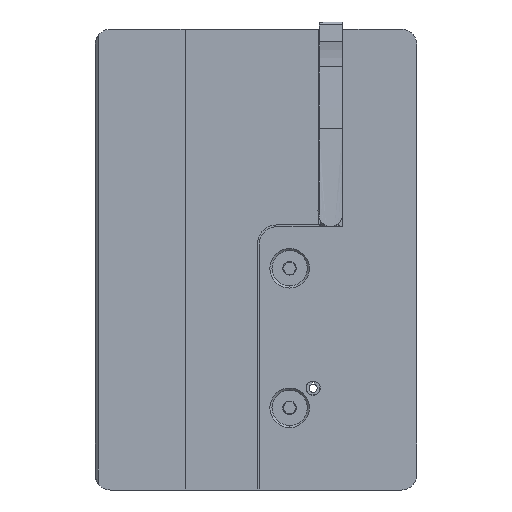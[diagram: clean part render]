
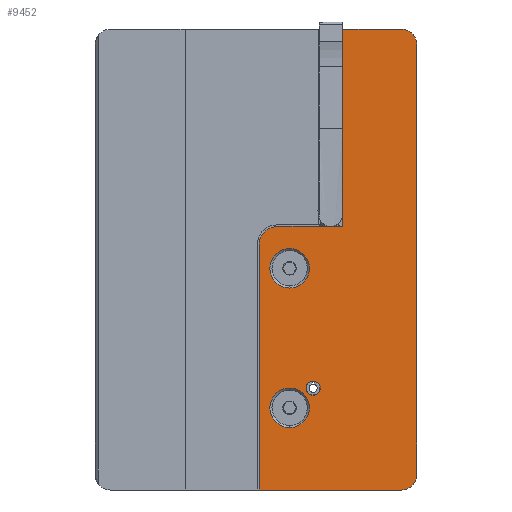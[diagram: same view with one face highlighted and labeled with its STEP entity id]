
A CAD part, left-side view. The second image highlights one B-rep face of the part: STEP entity #9452.
In plain terms, the highlighted planar face has unit normal (-1, 0, 0).
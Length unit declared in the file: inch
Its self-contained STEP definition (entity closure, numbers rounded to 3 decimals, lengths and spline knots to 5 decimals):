
#277 = CARTESIAN_POINT ( 'NONE',  ( -0.5, -0.41732, 0.025 ) ) ;
#498 = AXIS2_PLACEMENT_3D ( 'NONE', #7511, #19767, #10806 ) ;
#588 = EDGE_CURVE ( 'NONE', #7306, #6336, #9116, .T. ) ;
#1008 = CIRCLE ( 'NONE', #19829, 0.1 ) ;
#1064 = EDGE_CURVE ( 'NONE', #22464, #15260, #9641, .T. ) ;
#1150 = CARTESIAN_POINT ( 'NONE',  ( -0.5, 0.33268, -1.34272 ) ) ;
#1222 = CARTESIAN_POINT ( 'NONE',  ( -0.5, -0.51732, -2.85894 ) ) ;
#1831 = ORIENTED_EDGE ( 'NONE', *, *, #11971, .F. ) ;
#1925 = DIRECTION ( 'NONE',  ( -1., 0., 0. ) ) ;
#2478 = DIRECTION ( 'NONE',  ( 0., 0., 1. ) ) ;
#2717 = CARTESIAN_POINT ( 'NONE',  ( -0.5, 0.17531, -2.32502 ) ) ;
#2830 = PLANE ( 'NONE',  #10038 ) ;
#3038 = DIRECTION ( 'NONE',  ( -1., 0., 0. ) ) ;
#3093 = CARTESIAN_POINT ( 'NONE',  ( -0.5, 0.41187, -1.195 ) ) ;
#3456 = VERTEX_POINT ( 'NONE', #22065 ) ;
#3533 = EDGE_CURVE ( 'NONE', #13325, #19146, #14831, .T. ) ;
#3816 = DIRECTION ( 'NONE',  ( 0., 0., -1. ) ) ;
#3877 = CARTESIAN_POINT ( 'NONE',  ( -0.5, -0.51732, 0.125 ) ) ;
#4134 = CARTESIAN_POINT ( 'NONE',  ( -0.5, 0.53687, -1.195 ) ) ;
#4220 = DIRECTION ( 'NONE',  ( 0., 0., -1. ) ) ;
#4461 = ORIENTED_EDGE ( 'NONE', *, *, #13157, .F. ) ;
#4485 = DIRECTION ( 'NONE',  ( -1., 0., 0. ) ) ;
#4728 = ORIENTED_EDGE ( 'NONE', *, *, #16448, .F. ) ;
#5050 = VECTOR ( 'NONE', #4220, 39.37008 ) ;
#5121 = CARTESIAN_POINT ( 'NONE',  ( -0.5, -0.02313, 0.125 ) ) ;
#5163 = CARTESIAN_POINT ( 'NONE',  ( -0.5, 0.53687, -1.32 ) ) ;
#5471 = CARTESIAN_POINT ( 'NONE',  ( -0.5, -0.51732, 0.025 ) ) ;
#5515 = EDGE_CURVE ( 'NONE', #19146, #13325, #7239, .T. ) ;
#5532 = CARTESIAN_POINT ( 'NONE',  ( -0.5, 0.17531, -2.27752 ) ) ;
#5645 = DIRECTION ( 'NONE',  ( -1., 0., 0. ) ) ;
#5661 = AXIS2_PLACEMENT_3D ( 'NONE', #5532, #5645, #12807 ) ;
#5664 = LINE ( 'NONE', #12823, #6266 ) ;
#5711 = FACE_OUTER_BOUND ( 'NONE', #12936, .T. ) ;
#5741 = VERTEX_POINT ( 'NONE', #17261 ) ;
#6068 = VECTOR ( 'NONE', #6070, 39.37008 ) ;
#6070 = DIRECTION ( 'NONE',  ( 0., 1., 0. ) ) ;
#6266 = VECTOR ( 'NONE', #16481, 39.37008 ) ;
#6329 = DIRECTION ( 'NONE',  ( 0., 0., 1. ) ) ;
#6336 = VERTEX_POINT ( 'NONE', #1222 ) ;
#6407 = VERTEX_POINT ( 'NONE', #5471 ) ;
#6463 = FACE_BOUND ( 'NONE', #16546, .T. ) ;
#6827 = CIRCLE ( 'NONE', #8323, 0.13228 ) ;
#6839 = DIRECTION ( 'NONE',  ( -1., 0., 0. ) ) ;
#7117 = CIRCLE ( 'NONE', #19930, 0.0475 ) ;
#7217 = CARTESIAN_POINT ( 'NONE',  ( -0.5, 0.33268, -2.409 ) ) ;
#7239 = CIRCLE ( 'NONE', #498, 0.13228 ) ;
#7306 = VERTEX_POINT ( 'NONE', #19699 ) ;
#7511 = CARTESIAN_POINT ( 'NONE',  ( -0.5, 0.33268, -1.475 ) ) ;
#8208 = CARTESIAN_POINT ( 'NONE',  ( -0.5, 0.33268, -1.475 ) ) ;
#8210 = VERTEX_POINT ( 'NONE', #20801 ) ;
#8323 = AXIS2_PLACEMENT_3D ( 'NONE', #7217, #1925, #9099 ) ;
#8377 = EDGE_LOOP ( 'NONE', ( #10103, #8920 ) ) ;
#8915 = CARTESIAN_POINT ( 'NONE',  ( -0.5, -0.23642, 0.125 ) ) ;
#8920 = ORIENTED_EDGE ( 'NONE', *, *, #3533, .F. ) ;
#8970 = DIRECTION ( 'NONE',  ( 0., 0., -1. ) ) ;
#9099 = DIRECTION ( 'NONE',  ( 0., 0., 1. ) ) ;
#9116 = CIRCLE ( 'NONE', #11008, 0.1 ) ;
#9452 = ADVANCED_FACE ( 'NONE', ( #5711, #6463, #16952, #21830 ), #2830, .F. ) ;
#9533 = ORIENTED_EDGE ( 'NONE', *, *, #11877, .T. ) ;
#9641 = LINE ( 'NONE', #4134, #13998 ) ;
#10003 = DIRECTION ( 'NONE',  ( 1., 0., 0. ) ) ;
#10038 = AXIS2_PLACEMENT_3D ( 'NONE', #15413, #10003, #22475 ) ;
#10048 = CARTESIAN_POINT ( 'NONE',  ( -0.5, -0.02313, -1.195 ) ) ;
#10103 = ORIENTED_EDGE ( 'NONE', *, *, #5515, .F. ) ;
#10136 = CARTESIAN_POINT ( 'NONE',  ( -0.5, 0.17531, -2.23002 ) ) ;
#10483 = ORIENTED_EDGE ( 'NONE', *, *, #12620, .T. ) ;
#10503 = LINE ( 'NONE', #5121, #22251 ) ;
#10806 = DIRECTION ( 'NONE',  ( 0., 0., 1. ) ) ;
#11008 = AXIS2_PLACEMENT_3D ( 'NONE', #21718, #17941, #3816 ) ;
#11050 = LINE ( 'NONE', #3877, #5050 ) ;
#11057 = CARTESIAN_POINT ( 'NONE',  ( -0.5, 0.33268, -2.409 ) ) ;
#11141 = ORIENTED_EDGE ( 'NONE', *, *, #19686, .F. ) ;
#11406 = CARTESIAN_POINT ( 'NONE',  ( -0.5, -0.41732, 0.125 ) ) ;
#11481 = LINE ( 'NONE', #22310, #6068 ) ;
#11877 = EDGE_CURVE ( 'NONE', #22464, #17074, #18717, .T. ) ;
#11962 = EDGE_LOOP ( 'NONE', ( #15218, #17187 ) ) ;
#11971 = EDGE_CURVE ( 'NONE', #14764, #17074, #5664, .T. ) ;
#12027 = CIRCLE ( 'NONE', #5661, 0.0475 ) ;
#12370 = DIRECTION ( 'NONE',  ( 0., 0., 1. ) ) ;
#12620 = EDGE_CURVE ( 'NONE', #6407, #19960, #1008, .T. ) ;
#12807 = DIRECTION ( 'NONE',  ( 0., 0., 1. ) ) ;
#12823 = CARTESIAN_POINT ( 'NONE',  ( -0.5, 0.53687, -2.95894 ) ) ;
#12936 = EDGE_LOOP ( 'NONE', ( #20408, #21077, #4461, #10483, #16747, #11141, #20574, #9533, #1831 ) ) ;
#12940 = AXIS2_PLACEMENT_3D ( 'NONE', #8208, #3038, #6329 ) ;
#13065 = DIRECTION ( 'NONE',  ( 0., -1., 0. ) ) ;
#13157 = EDGE_CURVE ( 'NONE', #6407, #6336, #11050, .T. ) ;
#13325 = VERTEX_POINT ( 'NONE', #15236 ) ;
#13397 = AXIS2_PLACEMENT_3D ( 'NONE', #22236, #22018, #18123 ) ;
#13901 = VERTEX_POINT ( 'NONE', #10136 ) ;
#13998 = VECTOR ( 'NONE', #13065, 39.37008 ) ;
#14764 = VERTEX_POINT ( 'NONE', #15451 ) ;
#14831 = CIRCLE ( 'NONE', #12940, 0.13228 ) ;
#15078 = CIRCLE ( 'NONE', #19208, 0.13228 ) ;
#15218 = ORIENTED_EDGE ( 'NONE', *, *, #21934, .F. ) ;
#15236 = CARTESIAN_POINT ( 'NONE',  ( -0.5, 0.33268, -1.60728 ) ) ;
#15260 = VERTEX_POINT ( 'NONE', #10048 ) ;
#15413 = CARTESIAN_POINT ( 'NONE',  ( -0.5, 0., 0. ) ) ;
#15451 = CARTESIAN_POINT ( 'NONE',  ( -0.5, 0.53687, -2.95894 ) ) ;
#15996 = EDGE_CURVE ( 'NONE', #18796, #13901, #7117, .T. ) ;
#16095 = DIRECTION ( 'NONE',  ( 0., 1., 0. ) ) ;
#16448 = EDGE_CURVE ( 'NONE', #13901, #18796, #12027, .T. ) ;
#16481 = DIRECTION ( 'NONE',  ( 0., 0., 1. ) ) ;
#16546 = EDGE_LOOP ( 'NONE', ( #4728, #19377 ) ) ;
#16644 = VECTOR ( 'NONE', #16095, 39.37008 ) ;
#16747 = ORIENTED_EDGE ( 'NONE', *, *, #20383, .T. ) ;
#16952 = FACE_BOUND ( 'NONE', #11962, .T. ) ;
#17074 = VERTEX_POINT ( 'NONE', #5163 ) ;
#17187 = ORIENTED_EDGE ( 'NONE', *, *, #18343, .F. ) ;
#17261 = CARTESIAN_POINT ( 'NONE',  ( -0.5, -0.02313, 0.125 ) ) ;
#17744 = LINE ( 'NONE', #8915, #16644 ) ;
#17925 = DIRECTION ( 'NONE',  ( -1., 0., 0. ) ) ;
#17941 = DIRECTION ( 'NONE',  ( -1., 0., 0. ) ) ;
#18123 = DIRECTION ( 'NONE',  ( 0., 0., -1. ) ) ;
#18343 = EDGE_CURVE ( 'NONE', #8210, #3456, #15078, .T. ) ;
#18717 = CIRCLE ( 'NONE', #13397, 0.125 ) ;
#18796 = VERTEX_POINT ( 'NONE', #2717 ) ;
#19146 = VERTEX_POINT ( 'NONE', #1150 ) ;
#19208 = AXIS2_PLACEMENT_3D ( 'NONE', #11057, #6839, #12370 ) ;
#19377 = ORIENTED_EDGE ( 'NONE', *, *, #15996, .F. ) ;
#19686 = EDGE_CURVE ( 'NONE', #15260, #5741, #10503, .T. ) ;
#19699 = CARTESIAN_POINT ( 'NONE',  ( -0.5, -0.41732, -2.95894 ) ) ;
#19767 = DIRECTION ( 'NONE',  ( -1., 0., 0. ) ) ;
#19829 = AXIS2_PLACEMENT_3D ( 'NONE', #277, #17925, #8970 ) ;
#19930 = AXIS2_PLACEMENT_3D ( 'NONE', #20603, #4485, #2478 ) ;
#19960 = VERTEX_POINT ( 'NONE', #11406 ) ;
#20383 = EDGE_CURVE ( 'NONE', #19960, #5741, #17744, .T. ) ;
#20408 = ORIENTED_EDGE ( 'NONE', *, *, #21526, .F. ) ;
#20574 = ORIENTED_EDGE ( 'NONE', *, *, #1064, .F. ) ;
#20603 = CARTESIAN_POINT ( 'NONE',  ( -0.5, 0.17531, -2.27752 ) ) ;
#20801 = CARTESIAN_POINT ( 'NONE',  ( -0.5, 0.33268, -2.54128 ) ) ;
#21077 = ORIENTED_EDGE ( 'NONE', *, *, #588, .T. ) ;
#21526 = EDGE_CURVE ( 'NONE', #7306, #14764, #11481, .T. ) ;
#21718 = CARTESIAN_POINT ( 'NONE',  ( -0.5, -0.41732, -2.85894 ) ) ;
#21830 = FACE_BOUND ( 'NONE', #8377, .T. ) ;
#21934 = EDGE_CURVE ( 'NONE', #3456, #8210, #6827, .T. ) ;
#22018 = DIRECTION ( 'NONE',  ( -1., 0., 0. ) ) ;
#22065 = CARTESIAN_POINT ( 'NONE',  ( -0.5, 0.33268, -2.27672 ) ) ;
#22236 = CARTESIAN_POINT ( 'NONE',  ( -0.5, 0.41187, -1.32 ) ) ;
#22251 = VECTOR ( 'NONE', #23092, 39.37008 ) ;
#22310 = CARTESIAN_POINT ( 'NONE',  ( -0.5, -0.36732, -2.95894 ) ) ;
#22464 = VERTEX_POINT ( 'NONE', #3093 ) ;
#22475 = DIRECTION ( 'NONE',  ( 0., 0., -1. ) ) ;
#23092 = DIRECTION ( 'NONE',  ( 0., 0., 1. ) ) ;
